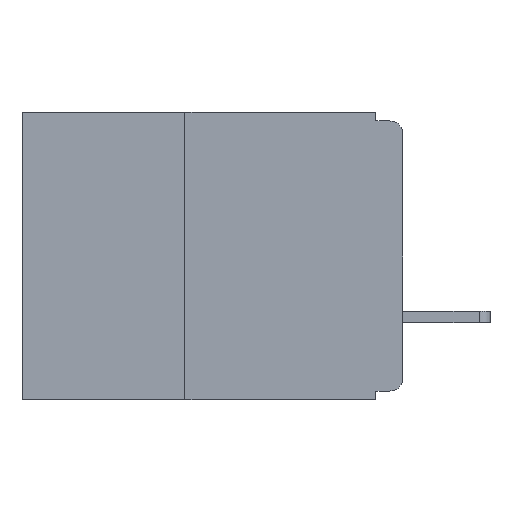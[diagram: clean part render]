
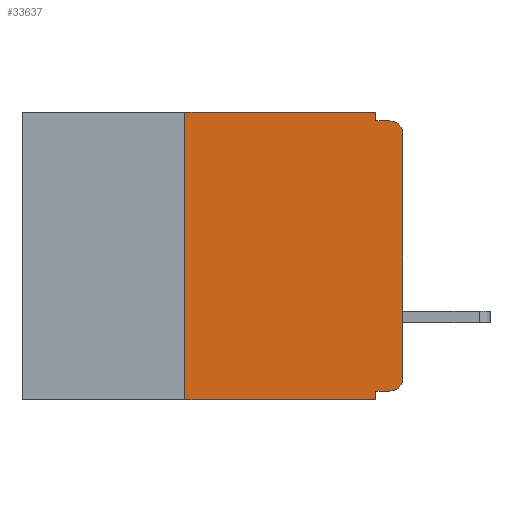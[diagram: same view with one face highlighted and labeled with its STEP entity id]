
A CAD part, left-side view. The second image highlights one B-rep face of the part: STEP entity #33637.
In plain terms, the highlighted planar face has unit normal (-1, 0, 0).
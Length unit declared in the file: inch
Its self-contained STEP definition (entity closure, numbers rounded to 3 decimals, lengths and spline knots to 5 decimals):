
#595 = CARTESIAN_POINT ( 'NONE',  ( 0., 0.015, -0.025 ) ) ;
#690 = LINE ( 'NONE', #28732, #27734 ) ;
#1516 = CARTESIAN_POINT ( 'NONE',  ( 0., 0.437, 0. ) ) ;
#1521 = CARTESIAN_POINT ( 'NONE',  ( 0., 0.25, 0. ) ) ;
#1590 = VERTEX_POINT ( 'NONE', #3528 ) ;
#1814 = LINE ( 'NONE', #31352, #20353 ) ;
#1983 = DIRECTION ( 'NONE',  ( 0., 0., 1. ) ) ;
#2015 = EDGE_CURVE ( 'NONE', #10936, #9349, #19635, .T. ) ;
#2237 = CARTESIAN_POINT ( 'NONE',  ( 0., 0.031, -0.33 ) ) ;
#2347 = DIRECTION ( 'NONE',  ( 0., 0., -1. ) ) ;
#2578 = DIRECTION ( 'NONE',  ( 0., -1., 0. ) ) ;
#3288 = DIRECTION ( 'NONE',  ( 0., 0., -1. ) ) ;
#3528 = CARTESIAN_POINT ( 'NONE',  ( 0., 0.25, -0.33 ) ) ;
#4228 = DIRECTION ( 'NONE',  ( 1., 0., 0. ) ) ;
#5886 = ORIENTED_EDGE ( 'NONE', *, *, #32172, .T. ) ;
#6248 = ORIENTED_EDGE ( 'NONE', *, *, #11587, .F. ) ;
#6587 = VERTEX_POINT ( 'NONE', #22349 ) ;
#6815 = DIRECTION ( 'NONE',  ( 0., -1., 0. ) ) ;
#8714 = AXIS2_PLACEMENT_3D ( 'NONE', #1516, #4228, #22536 ) ;
#9349 = VERTEX_POINT ( 'NONE', #23198 ) ;
#9640 = EDGE_CURVE ( 'NONE', #16825, #10936, #25291, .T. ) ;
#10045 = VECTOR ( 'NONE', #10320, 39.37008 ) ;
#10187 = VECTOR ( 'NONE', #2347, 39.37008 ) ;
#10320 = DIRECTION ( 'NONE',  ( 0., -1., 0. ) ) ;
#10936 = VERTEX_POINT ( 'NONE', #25495 ) ;
#11544 = LINE ( 'NONE', #33963, #16872 ) ;
#11587 = EDGE_CURVE ( 'NONE', #17806, #11993, #20333, .T. ) ;
#11803 = VECTOR ( 'NONE', #2578, 39.37008 ) ;
#11993 = VERTEX_POINT ( 'NONE', #30431 ) ;
#12944 = CARTESIAN_POINT ( 'NONE',  ( 0., 0.031, 0. ) ) ;
#13395 = CARTESIAN_POINT ( 'NONE',  ( 0., 0.015, -0.305 ) ) ;
#14714 = ORIENTED_EDGE ( 'NONE', *, *, #16273, .T. ) ;
#15007 = CIRCLE ( 'NONE', #31772, 0.015 ) ;
#16031 = DIRECTION ( 'NONE',  ( 0., 0., -1. ) ) ;
#16273 = EDGE_CURVE ( 'NONE', #1590, #16888, #1814, .T. ) ;
#16399 = LINE ( 'NONE', #2237, #10187 ) ;
#16825 = VERTEX_POINT ( 'NONE', #31086 ) ;
#16872 = VECTOR ( 'NONE', #28717, 39.37008 ) ;
#16888 = VERTEX_POINT ( 'NONE', #23595 ) ;
#17806 = VERTEX_POINT ( 'NONE', #1521 ) ;
#17851 = CARTESIAN_POINT ( 'NONE',  ( 0., 0., 0. ) ) ;
#18314 = ORIENTED_EDGE ( 'NONE', *, *, #25538, .F. ) ;
#19066 = DIRECTION ( 'NONE',  ( -1., 0., 0. ) ) ;
#19635 = CIRCLE ( 'NONE', #29986, 0.015 ) ;
#19864 = ORIENTED_EDGE ( 'NONE', *, *, #2015, .T. ) ;
#20333 = LINE ( 'NONE', #28650, #11803 ) ;
#20353 = VECTOR ( 'NONE', #6815, 39.37008 ) ;
#20632 = DIRECTION ( 'NONE',  ( 0., 0., -1. ) ) ;
#20855 = EDGE_CURVE ( 'NONE', #6587, #25667, #11544, .T. ) ;
#21315 = CARTESIAN_POINT ( 'NONE',  ( 0., 0.031, -0.32 ) ) ;
#21322 = EDGE_CURVE ( 'NONE', #33305, #9349, #30751, .T. ) ;
#21942 = EDGE_CURVE ( 'NONE', #11993, #33305, #23863, .T. ) ;
#22163 = ORIENTED_EDGE ( 'NONE', *, *, #24345, .F. ) ;
#22349 = CARTESIAN_POINT ( 'NONE',  ( 0., 0.015, -0.32 ) ) ;
#22536 = DIRECTION ( 'NONE',  ( 0., 0., -1. ) ) ;
#22741 = ORIENTED_EDGE ( 'NONE', *, *, #21322, .F. ) ;
#23198 = CARTESIAN_POINT ( 'NONE',  ( 0., 0.015, -0.01 ) ) ;
#23595 = CARTESIAN_POINT ( 'NONE',  ( 0., 0.031, -0.33 ) ) ;
#23863 = LINE ( 'NONE', #12944, #29939 ) ;
#24345 = EDGE_CURVE ( 'NONE', #1590, #17806, #690, .T. ) ;
#25291 = LINE ( 'NONE', #17851, #30562 ) ;
#25495 = CARTESIAN_POINT ( 'NONE',  ( 0., 0., -0.025 ) ) ;
#25538 = EDGE_CURVE ( 'NONE', #25667, #16888, #16399, .T. ) ;
#25667 = VERTEX_POINT ( 'NONE', #21315 ) ;
#26397 = CARTESIAN_POINT ( 'NONE',  ( 0., 0.031, -0.01 ) ) ;
#26568 = EDGE_LOOP ( 'NONE', ( #29613, #19864, #22741, #30650, #6248, #22163, #14714, #18314, #31379, #5886 ) ) ;
#27734 = VECTOR ( 'NONE', #31337, 39.37008 ) ;
#28650 = CARTESIAN_POINT ( 'NONE',  ( 0., 0.437, 0. ) ) ;
#28717 = DIRECTION ( 'NONE',  ( 0., 1., 0. ) ) ;
#28732 = CARTESIAN_POINT ( 'NONE',  ( 0., 0.25, -0.33 ) ) ;
#29059 = FACE_OUTER_BOUND ( 'NONE', #26568, .T. ) ;
#29613 = ORIENTED_EDGE ( 'NONE', *, *, #9640, .T. ) ;
#29939 = VECTOR ( 'NONE', #20632, 39.37008 ) ;
#29986 = AXIS2_PLACEMENT_3D ( 'NONE', #595, #19066, #3288 ) ;
#30431 = CARTESIAN_POINT ( 'NONE',  ( 0., 0.031, 0. ) ) ;
#30562 = VECTOR ( 'NONE', #1983, 39.37008 ) ;
#30650 = ORIENTED_EDGE ( 'NONE', *, *, #21942, .F. ) ;
#30751 = LINE ( 'NONE', #33604, #10045 ) ;
#31086 = CARTESIAN_POINT ( 'NONE',  ( 0., 0., -0.305 ) ) ;
#31337 = DIRECTION ( 'NONE',  ( 0., 0., 1. ) ) ;
#31352 = CARTESIAN_POINT ( 'NONE',  ( 0., 0.437, -0.33 ) ) ;
#31379 = ORIENTED_EDGE ( 'NONE', *, *, #20855, .F. ) ;
#31473 = DIRECTION ( 'NONE',  ( -1., 0., 0. ) ) ;
#31772 = AXIS2_PLACEMENT_3D ( 'NONE', #13395, #31473, #16031 ) ;
#32172 = EDGE_CURVE ( 'NONE', #6587, #16825, #15007, .T. ) ;
#32867 = PLANE ( 'NONE',  #8714 ) ;
#33305 = VERTEX_POINT ( 'NONE', #26397 ) ;
#33604 = CARTESIAN_POINT ( 'NONE',  ( 0., 0., -0.01 ) ) ;
#33637 = ADVANCED_FACE ( 'NONE', ( #29059 ), #32867, .F. ) ;
#33963 = CARTESIAN_POINT ( 'NONE',  ( 0., 0., -0.32 ) ) ;
